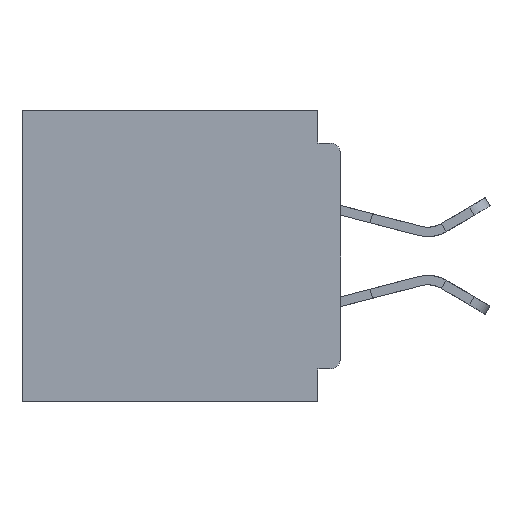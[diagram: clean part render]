
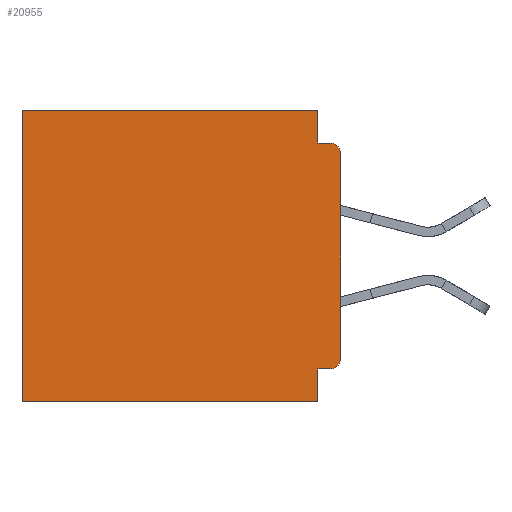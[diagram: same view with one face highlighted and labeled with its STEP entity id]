
A CAD part, left-side view. The second image highlights one B-rep face of the part: STEP entity #20955.
In plain terms, the highlighted planar face has unit normal (-1, 0, 0).
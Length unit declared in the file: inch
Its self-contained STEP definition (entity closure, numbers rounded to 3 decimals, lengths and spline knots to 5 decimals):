
#499 = ORIENTED_EDGE ( 'NONE', *, *, #42657, .T. ) ;
#1497 = EDGE_CURVE ( 'NONE', #32127, #18696, #29962, .T. ) ;
#1666 = ORIENTED_EDGE ( 'NONE', *, *, #1497, .T. ) ;
#2523 = CARTESIAN_POINT ( 'NONE',  ( 0.3, 0.015, -0.06 ) ) ;
#4259 = EDGE_CURVE ( 'NONE', #26509, #30920, #8542, .T. ) ;
#4987 = CARTESIAN_POINT ( 'NONE',  ( 0.3, 0., -0.4 ) ) ;
#5570 = ORIENTED_EDGE ( 'NONE', *, *, #4259, .T. ) ;
#5980 = DIRECTION ( 'NONE',  ( 0., 0., -1. ) ) ;
#6593 = EDGE_CURVE ( 'NONE', #43086, #18696, #16198, .T. ) ;
#6970 = ORIENTED_EDGE ( 'NONE', *, *, #8136, .F. ) ;
#7575 = LINE ( 'NONE', #4987, #16487 ) ;
#8136 = EDGE_CURVE ( 'NONE', #14857, #43086, #10816, .T. ) ;
#8200 = CARTESIAN_POINT ( 'NONE',  ( 0.3, 0.015, -0.34 ) ) ;
#8542 = CIRCLE ( 'NONE', #15090, 0.015 ) ;
#8723 = VECTOR ( 'NONE', #10438, 39.37008 ) ;
#8998 = EDGE_LOOP ( 'NONE', ( #24049, #43468, #37569, #37108, #499, #1666, #41948, #6970, #23262, #5570 ) ) ;
#10010 = CARTESIAN_POINT ( 'NONE',  ( 0.3, 0., -0.045 ) ) ;
#10438 = DIRECTION ( 'NONE',  ( 0., 0., -1. ) ) ;
#10816 = LINE ( 'NONE', #33869, #8723 ) ;
#11192 = EDGE_CURVE ( 'NONE', #16455, #30920, #7575, .T. ) ;
#11555 = DIRECTION ( 'NONE',  ( 0., 0., -1. ) ) ;
#12320 = FACE_OUTER_BOUND ( 'NONE', #8998, .T. ) ;
#13384 = DIRECTION ( 'NONE',  ( 0., -1., 0. ) ) ;
#13608 = CARTESIAN_POINT ( 'NONE',  ( 0.3, 0., -0.4 ) ) ;
#13771 = DIRECTION ( 'NONE',  ( 0., 0., -1. ) ) ;
#14713 = VECTOR ( 'NONE', #23033, 39.37008 ) ;
#14857 = VERTEX_POINT ( 'NONE', #32132 ) ;
#14986 = DIRECTION ( 'NONE',  ( 0., 0., -1. ) ) ;
#15090 = AXIS2_PLACEMENT_3D ( 'NONE', #8200, #31649, #11555 ) ;
#16198 = LINE ( 'NONE', #24028, #41837 ) ;
#16455 = VERTEX_POINT ( 'NONE', #21328 ) ;
#16487 = VECTOR ( 'NONE', #14986, 39.37008 ) ;
#16664 = VECTOR ( 'NONE', #31240, 39.37008 ) ;
#17555 = DIRECTION ( 'NONE',  ( 0., 1., 0. ) ) ;
#18696 = VERTEX_POINT ( 'NONE', #24831 ) ;
#18963 = CARTESIAN_POINT ( 'NONE',  ( 0.3, 0.031, 0. ) ) ;
#19073 = AXIS2_PLACEMENT_3D ( 'NONE', #13608, #33825, #13771 ) ;
#20955 = ADVANCED_FACE ( 'NONE', ( #12320 ), #30477, .F. ) ;
#21063 = VECTOR ( 'NONE', #28929, 39.37008 ) ;
#21131 = CIRCLE ( 'NONE', #21248, 0.015 ) ;
#21248 = AXIS2_PLACEMENT_3D ( 'NONE', #2523, #26101, #5980 ) ;
#21328 = CARTESIAN_POINT ( 'NONE',  ( 0.3, 0., -0.06 ) ) ;
#21978 = VERTEX_POINT ( 'NONE', #38702 ) ;
#22286 = LINE ( 'NONE', #26526, #38967 ) ;
#23033 = DIRECTION ( 'NONE',  ( 0., 0., -1. ) ) ;
#23262 = ORIENTED_EDGE ( 'NONE', *, *, #38468, .F. ) ;
#24028 = CARTESIAN_POINT ( 'NONE',  ( 0.3, 0., -0.4 ) ) ;
#24049 = ORIENTED_EDGE ( 'NONE', *, *, #11192, .F. ) ;
#24086 = EDGE_CURVE ( 'NONE', #37649, #21978, #24704, .T. ) ;
#24704 = LINE ( 'NONE', #39653, #14713 ) ;
#24831 = CARTESIAN_POINT ( 'NONE',  ( 0.3, 0.437, -0.4 ) ) ;
#25185 = LINE ( 'NONE', #10010, #42895 ) ;
#26101 = DIRECTION ( 'NONE',  ( -1., 0., 0. ) ) ;
#26509 = VERTEX_POINT ( 'NONE', #32794 ) ;
#26526 = CARTESIAN_POINT ( 'NONE',  ( 0.3, 0., -0.355 ) ) ;
#28621 = EDGE_CURVE ( 'NONE', #16455, #31969, #21131, .T. ) ;
#28929 = DIRECTION ( 'NONE',  ( 0., 0., -1. ) ) ;
#29859 = DIRECTION ( 'NONE',  ( 0., 1., 0. ) ) ;
#29962 = LINE ( 'NONE', #30913, #21063 ) ;
#30314 = CARTESIAN_POINT ( 'NONE',  ( 0.3, 0.031, -0.4 ) ) ;
#30477 = PLANE ( 'NONE',  #19073 ) ;
#30611 = CARTESIAN_POINT ( 'NONE',  ( 0.3, 0.015, -0.045 ) ) ;
#30913 = CARTESIAN_POINT ( 'NONE',  ( 0.3, 0.437, -0.4 ) ) ;
#30920 = VERTEX_POINT ( 'NONE', #35478 ) ;
#31240 = DIRECTION ( 'NONE',  ( 0., 1., 0. ) ) ;
#31649 = DIRECTION ( 'NONE',  ( -1., 0., 0. ) ) ;
#31969 = VERTEX_POINT ( 'NONE', #30611 ) ;
#32127 = VERTEX_POINT ( 'NONE', #34652 ) ;
#32132 = CARTESIAN_POINT ( 'NONE',  ( 0.3, 0.031, -0.355 ) ) ;
#32794 = CARTESIAN_POINT ( 'NONE',  ( 0.3, 0.015, -0.355 ) ) ;
#33799 = EDGE_CURVE ( 'NONE', #21978, #31969, #25185, .T. ) ;
#33825 = DIRECTION ( 'NONE',  ( 1., 0., 0. ) ) ;
#33869 = CARTESIAN_POINT ( 'NONE',  ( 0.3, 0.031, -0.4 ) ) ;
#34439 = LINE ( 'NONE', #37784, #16664 ) ;
#34652 = CARTESIAN_POINT ( 'NONE',  ( 0.3, 0.437, 0. ) ) ;
#35478 = CARTESIAN_POINT ( 'NONE',  ( 0.3, 0., -0.34 ) ) ;
#37108 = ORIENTED_EDGE ( 'NONE', *, *, #24086, .F. ) ;
#37569 = ORIENTED_EDGE ( 'NONE', *, *, #33799, .F. ) ;
#37649 = VERTEX_POINT ( 'NONE', #18963 ) ;
#37784 = CARTESIAN_POINT ( 'NONE',  ( 0.3, 0., 0. ) ) ;
#38468 = EDGE_CURVE ( 'NONE', #26509, #14857, #22286, .T. ) ;
#38702 = CARTESIAN_POINT ( 'NONE',  ( 0.3, 0.031, -0.045 ) ) ;
#38967 = VECTOR ( 'NONE', #29859, 39.37008 ) ;
#39653 = CARTESIAN_POINT ( 'NONE',  ( 0.3, 0.031, 0. ) ) ;
#41837 = VECTOR ( 'NONE', #17555, 39.37008 ) ;
#41948 = ORIENTED_EDGE ( 'NONE', *, *, #6593, .F. ) ;
#42657 = EDGE_CURVE ( 'NONE', #37649, #32127, #34439, .T. ) ;
#42895 = VECTOR ( 'NONE', #13384, 39.37008 ) ;
#43086 = VERTEX_POINT ( 'NONE', #30314 ) ;
#43468 = ORIENTED_EDGE ( 'NONE', *, *, #28621, .T. ) ;
